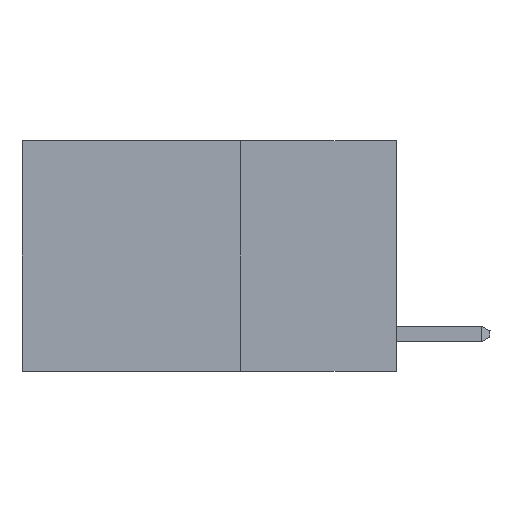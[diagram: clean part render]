
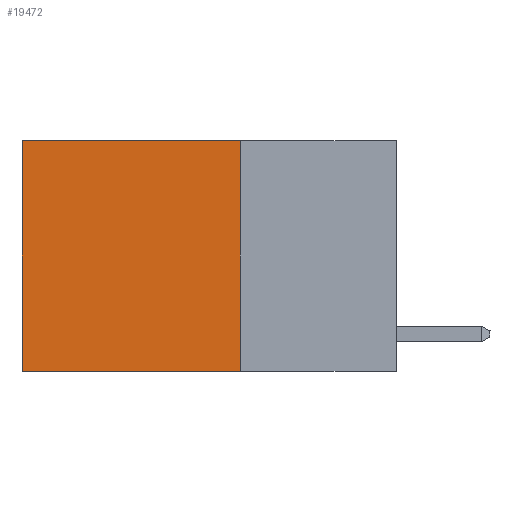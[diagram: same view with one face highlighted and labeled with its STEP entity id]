
A CAD part, left-side view. The second image highlights one B-rep face of the part: STEP entity #19472.
In plain terms, the highlighted planar face has unit normal (-1, 0, 0).
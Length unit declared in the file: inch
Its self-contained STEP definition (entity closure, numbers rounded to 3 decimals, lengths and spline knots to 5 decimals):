
#2267 = ORIENTED_EDGE ( 'NONE', *, *, #14727, .F. ) ;
#2812 = VERTEX_POINT ( 'NONE', #4911 ) ;
#4156 = AXIS2_PLACEMENT_3D ( 'NONE', #21062, #7623, #21146 ) ;
#4494 = EDGE_LOOP ( 'NONE', ( #8553, #2267, #20952, #4964 ) ) ;
#4660 = EDGE_CURVE ( 'NONE', #2812, #21794, #8425, .T. ) ;
#4911 = CARTESIAN_POINT ( 'NONE',  ( 0.2625, 0.6, 0. ) ) ;
#4964 = ORIENTED_EDGE ( 'NONE', *, *, #23742, .T. ) ;
#5834 = CARTESIAN_POINT ( 'NONE',  ( 0.2625, 0.25, 0. ) ) ;
#6882 = CARTESIAN_POINT ( 'NONE',  ( 0.2625, 0.25, 0. ) ) ;
#6929 = VECTOR ( 'NONE', #9269, 39.37008 ) ;
#7338 = CARTESIAN_POINT ( 'NONE',  ( 0.2625, 0.25, 0. ) ) ;
#7623 = DIRECTION ( 'NONE',  ( 1., 0., 0. ) ) ;
#8306 = CARTESIAN_POINT ( 'NONE',  ( 0.2625, 0.6, -0.37 ) ) ;
#8425 = LINE ( 'NONE', #14590, #13602 ) ;
#8553 = ORIENTED_EDGE ( 'NONE', *, *, #4660, .T. ) ;
#8739 = LINE ( 'NONE', #5834, #18439 ) ;
#9269 = DIRECTION ( 'NONE',  ( 0., 0., -1. ) ) ;
#9982 = CARTESIAN_POINT ( 'NONE',  ( 0.2625, 0.25, -0.37 ) ) ;
#11574 = VERTEX_POINT ( 'NONE', #16636 ) ;
#11949 = DIRECTION ( 'NONE',  ( 0., 1., 0. ) ) ;
#13573 = DIRECTION ( 'NONE',  ( 0., 1., 0. ) ) ;
#13602 = VECTOR ( 'NONE', #24199, 39.37008 ) ;
#14590 = CARTESIAN_POINT ( 'NONE',  ( 0.2625, 0.6, 0. ) ) ;
#14727 = EDGE_CURVE ( 'NONE', #11574, #21794, #15038, .T. ) ;
#15038 = LINE ( 'NONE', #9982, #18949 ) ;
#16636 = CARTESIAN_POINT ( 'NONE',  ( 0.2625, 0.25, -0.37 ) ) ;
#17237 = LINE ( 'NONE', #7338, #6929 ) ;
#18439 = VECTOR ( 'NONE', #13573, 39.37008 ) ;
#18949 = VECTOR ( 'NONE', #11949, 39.37008 ) ;
#19198 = PLANE ( 'NONE',  #4156 ) ;
#19254 = VERTEX_POINT ( 'NONE', #6882 ) ;
#19472 = ADVANCED_FACE ( 'NONE', ( #23843 ), #19198, .F. ) ;
#19976 = EDGE_CURVE ( 'NONE', #19254, #11574, #17237, .T. ) ;
#20952 = ORIENTED_EDGE ( 'NONE', *, *, #19976, .F. ) ;
#21062 = CARTESIAN_POINT ( 'NONE',  ( 0.2625, 0.25, 0. ) ) ;
#21146 = DIRECTION ( 'NONE',  ( 0., 0., -1. ) ) ;
#21794 = VERTEX_POINT ( 'NONE', #8306 ) ;
#23742 = EDGE_CURVE ( 'NONE', #19254, #2812, #8739, .T. ) ;
#23843 = FACE_OUTER_BOUND ( 'NONE', #4494, .T. ) ;
#24199 = DIRECTION ( 'NONE',  ( 0., 0., -1. ) ) ;
